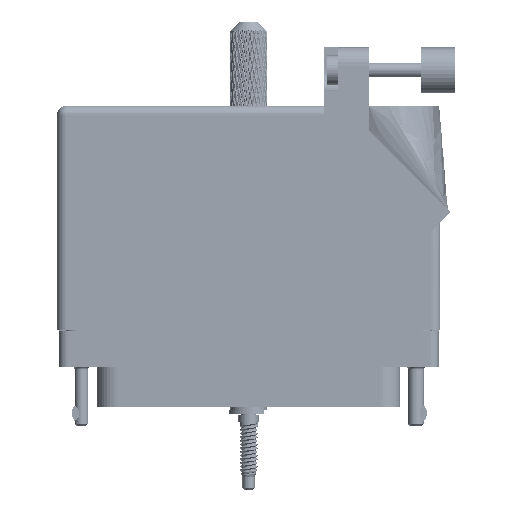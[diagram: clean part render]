
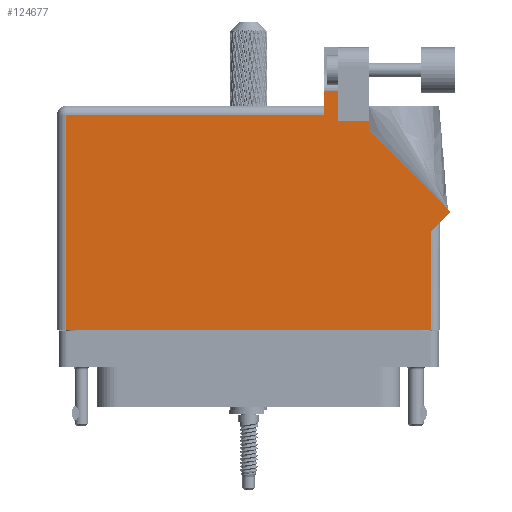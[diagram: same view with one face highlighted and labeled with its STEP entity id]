
A CAD part, front view. The second image highlights one B-rep face of the part: STEP entity #124677.
In plain terms, the highlighted face is planar.
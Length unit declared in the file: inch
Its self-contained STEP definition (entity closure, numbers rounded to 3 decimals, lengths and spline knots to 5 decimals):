
#264 = VERTEX_POINT ( 'NONE', #31390 ) ;
#3875 = ORIENTED_EDGE ( 'NONE', *, *, #93444, .T. ) ;
#5439 = CARTESIAN_POINT ( 'NONE',  ( -1.306, 1.368, 0.455 ) ) ;
#5533 = ORIENTED_EDGE ( 'NONE', *, *, #49963, .T. ) ;
#6732 = VERTEX_POINT ( 'NONE', #100201 ) ;
#9903 = DIRECTION ( 'NONE',  ( 0., 1., 0. ) ) ;
#9939 = CARTESIAN_POINT ( 'NONE',  ( 0.93777, 1.5315, 0.455 ) ) ;
#11118 = VERTEX_POINT ( 'NONE', #62886 ) ;
#12938 = LINE ( 'NONE', #9939, #25323 ) ;
#13564 = EDGE_CURVE ( 'NONE', #55092, #117915, #27199, .T. ) ;
#14683 = VERTEX_POINT ( 'NONE', #35460 ) ;
#16949 = EDGE_LOOP ( 'NONE', ( #19374, #3875, #98243, #117524, #5533, #104117, #116498, #107350, #53657, #127078, #87808 ) ) ;
#17194 = EDGE_CURVE ( 'NONE', #117915, #6732, #73972, .T. ) ;
#19374 = ORIENTED_EDGE ( 'NONE', *, *, #59094, .T. ) ;
#19833 = VECTOR ( 'NONE', #28611, 39.37008 ) ;
#20126 = LINE ( 'NONE', #43435, #75210 ) ;
#21447 = CARTESIAN_POINT ( 'NONE',  ( 1.244, 0.575, 0.455 ) ) ;
#22910 = VERTEX_POINT ( 'NONE', #95893 ) ;
#23771 = VERTEX_POINT ( 'NONE', #29300 ) ;
#25314 = CARTESIAN_POINT ( 'NONE',  ( 1.37671, 0.70771, 0.455 ) ) ;
#25323 = VECTOR ( 'NONE', #50221, 39.37008 ) ;
#27199 = LINE ( 'NONE', #58702, #76146 ) ;
#28558 = PLANE ( 'NONE',  #106325 ) ;
#28611 = DIRECTION ( 'NONE',  ( 0., 1., 0. ) ) ;
#29300 = CARTESIAN_POINT ( 'NONE',  ( 1.37671, 0.70771, 0.455 ) ) ;
#29887 = VECTOR ( 'NONE', #67982, 39.37008 ) ;
#30207 = VERTEX_POINT ( 'NONE', #98720 ) ;
#31390 = CARTESIAN_POINT ( 'NONE',  ( 0.513, 1.5315, 0.455 ) ) ;
#32368 = DIRECTION ( 'NONE',  ( 0.707, 0.707, 0. ) ) ;
#32639 = LINE ( 'NONE', #89737, #47972 ) ;
#32799 = CARTESIAN_POINT ( 'NONE',  ( 1.306, 0.637, 0.455 ) ) ;
#35460 = CARTESIAN_POINT ( 'NONE',  ( -1.244, 1.368, 0.455 ) ) ;
#39472 = CARTESIAN_POINT ( 'NONE',  ( 0.82, 1.33, 0.455 ) ) ;
#43435 = CARTESIAN_POINT ( 'NONE',  ( -1.306, -0.1, 0.455 ) ) ;
#44058 = DIRECTION ( 'NONE',  ( -0.707, 0.707, 0. ) ) ;
#46117 = DIRECTION ( 'NONE',  ( -1., 0., 0. ) ) ;
#47914 = VECTOR ( 'NONE', #71663, 39.37008 ) ;
#47972 = VECTOR ( 'NONE', #91017, 39.37008 ) ;
#49963 = EDGE_CURVE ( 'NONE', #14683, #101635, #32639, .T. ) ;
#50221 = DIRECTION ( 'NONE',  ( -1., 0., 0. ) ) ;
#50719 = LINE ( 'NONE', #5439, #110533 ) ;
#53256 = DIRECTION ( 'NONE',  ( 1., 0., 0. ) ) ;
#53657 = ORIENTED_EDGE ( 'NONE', *, *, #122351, .T. ) ;
#54539 = CARTESIAN_POINT ( 'NONE',  ( 0.82, 1.33, 0.455 ) ) ;
#55092 = VERTEX_POINT ( 'NONE', #85358 ) ;
#56957 = VECTOR ( 'NONE', #32368, 39.37008 ) ;
#57981 = CARTESIAN_POINT ( 'NONE',  ( -1.306, 1.43, 0.455 ) ) ;
#58702 = CARTESIAN_POINT ( 'NONE',  ( 0.82, 1.26442, 0.455 ) ) ;
#59094 = EDGE_CURVE ( 'NONE', #6732, #11118, #81988, .T. ) ;
#61127 = LINE ( 'NONE', #25314, #118100 ) ;
#62886 = CARTESIAN_POINT ( 'NONE',  ( 0.607, 1.5315, 0.455 ) ) ;
#67965 = CARTESIAN_POINT ( 'NONE',  ( 0.513, 1.43, 0.455 ) ) ;
#67982 = DIRECTION ( 'NONE',  ( 0., 1., 0. ) ) ;
#68524 = EDGE_CURVE ( 'NONE', #22910, #14683, #50719, .T. ) ;
#69867 = EDGE_CURVE ( 'NONE', #30207, #102878, #91855, .T. ) ;
#71663 = DIRECTION ( 'NONE',  ( -1., 0., 0. ) ) ;
#73059 = LINE ( 'NONE', #67965, #103771 ) ;
#73972 = LINE ( 'NONE', #54539, #47914 ) ;
#75210 = VECTOR ( 'NONE', #53256, 39.37008 ) ;
#76146 = VECTOR ( 'NONE', #9903, 39.37008 ) ;
#81988 = LINE ( 'NONE', #117007, #29887 ) ;
#84320 = CARTESIAN_POINT ( 'NONE',  ( -1.244, -0.1, 0.455 ) ) ;
#85358 = CARTESIAN_POINT ( 'NONE',  ( 0.82, 1.26442, 0.455 ) ) ;
#87808 = ORIENTED_EDGE ( 'NONE', *, *, #17194, .T. ) ;
#87813 = DIRECTION ( 'NONE',  ( 0., -1., 0. ) ) ;
#89737 = CARTESIAN_POINT ( 'NONE',  ( -1.244, -0.1, 0.455 ) ) ;
#91017 = DIRECTION ( 'NONE',  ( 0., -1., 0. ) ) ;
#91855 = LINE ( 'NONE', #116026, #19833 ) ;
#93444 = EDGE_CURVE ( 'NONE', #11118, #264, #12938, .T. ) ;
#95560 = FACE_OUTER_BOUND ( 'NONE', #16949, .T. ) ;
#95893 = CARTESIAN_POINT ( 'NONE',  ( 0.513, 1.368, 0.455 ) ) ;
#98243 = ORIENTED_EDGE ( 'NONE', *, *, #101615, .T. ) ;
#98720 = CARTESIAN_POINT ( 'NONE',  ( 1.244, -0.1, 0.455 ) ) ;
#99947 = DIRECTION ( 'NONE',  ( 0., 0., -1. ) ) ;
#100201 = CARTESIAN_POINT ( 'NONE',  ( 0.607, 1.33, 0.455 ) ) ;
#101615 = EDGE_CURVE ( 'NONE', #264, #22910, #73059, .T. ) ;
#101635 = VERTEX_POINT ( 'NONE', #84320 ) ;
#102878 = VERTEX_POINT ( 'NONE', #21447 ) ;
#103370 = EDGE_CURVE ( 'NONE', #102878, #23771, #116899, .T. ) ;
#103771 = VECTOR ( 'NONE', #87813, 39.37008 ) ;
#104117 = ORIENTED_EDGE ( 'NONE', *, *, #127059, .T. ) ;
#106325 = AXIS2_PLACEMENT_3D ( 'NONE', #57981, #99947, #110194 ) ;
#107350 = ORIENTED_EDGE ( 'NONE', *, *, #103370, .T. ) ;
#110194 = DIRECTION ( 'NONE',  ( -1., 0., 0. ) ) ;
#110533 = VECTOR ( 'NONE', #46117, 39.37008 ) ;
#116026 = CARTESIAN_POINT ( 'NONE',  ( 1.244, 0.637, 0.455 ) ) ;
#116498 = ORIENTED_EDGE ( 'NONE', *, *, #69867, .T. ) ;
#116899 = LINE ( 'NONE', #32799, #56957 ) ;
#117007 = CARTESIAN_POINT ( 'NONE',  ( 0.607, 1.33, 0.455 ) ) ;
#117524 = ORIENTED_EDGE ( 'NONE', *, *, #68524, .T. ) ;
#117915 = VERTEX_POINT ( 'NONE', #39472 ) ;
#118100 = VECTOR ( 'NONE', #44058, 39.37008 ) ;
#122351 = EDGE_CURVE ( 'NONE', #23771, #55092, #61127, .T. ) ;
#124677 = ADVANCED_FACE ( 'NONE', ( #95560 ), #28558, .F. ) ;
#127059 = EDGE_CURVE ( 'NONE', #101635, #30207, #20126, .T. ) ;
#127078 = ORIENTED_EDGE ( 'NONE', *, *, #13564, .T. ) ;
